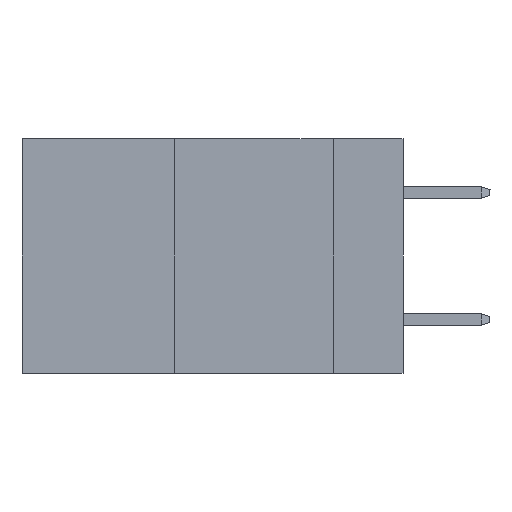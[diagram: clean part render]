
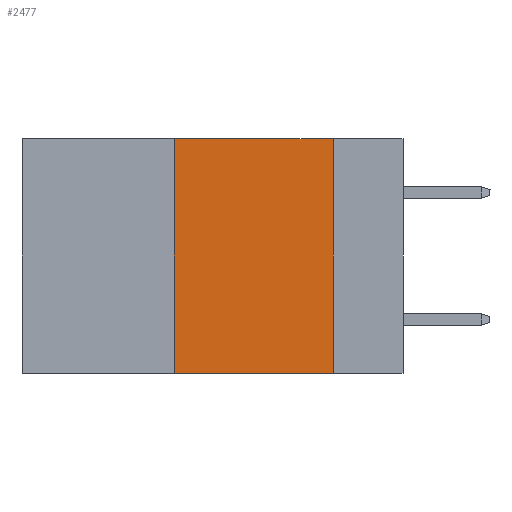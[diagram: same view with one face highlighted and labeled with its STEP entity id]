
A CAD part, left-side view. The second image highlights one B-rep face of the part: STEP entity #2477.
In plain terms, the highlighted planar face has unit normal (-1, 0, 0).
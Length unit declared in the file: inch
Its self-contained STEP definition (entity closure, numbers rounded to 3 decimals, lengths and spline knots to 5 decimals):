
#1628 = VERTEX_POINT ( 'NONE', #3738 ) ;
#1872 = EDGE_CURVE ( 'NONE', #18165, #4115, #6890, .T. ) ;
#2121 = ORIENTED_EDGE ( 'NONE', *, *, #6754, .F. ) ;
#2318 = EDGE_CURVE ( 'NONE', #18165, #10822, #6518, .T. ) ;
#2477 = ADVANCED_FACE ( 'NONE', ( #14035 ), #21450, .F. ) ;
#2865 = DIRECTION ( 'NONE',  ( 0., 0., -1. ) ) ;
#3508 = ORIENTED_EDGE ( 'NONE', *, *, #2318, .T. ) ;
#3557 = DIRECTION ( 'NONE',  ( 1., 0., 0. ) ) ;
#3738 = CARTESIAN_POINT ( 'NONE',  ( 0., 0.11, 0. ) ) ;
#4115 = VERTEX_POINT ( 'NONE', #4663 ) ;
#4663 = CARTESIAN_POINT ( 'NONE',  ( 0., 0.36, 0. ) ) ;
#4844 = LINE ( 'NONE', #12370, #21093 ) ;
#6518 = LINE ( 'NONE', #13802, #6992 ) ;
#6754 = EDGE_CURVE ( 'NONE', #4115, #1628, #4844, .T. ) ;
#6756 = VECTOR ( 'NONE', #2865, 39.37008 ) ;
#6890 = LINE ( 'NONE', #8611, #8922 ) ;
#6992 = VECTOR ( 'NONE', #17912, 39.37008 ) ;
#8611 = CARTESIAN_POINT ( 'NONE',  ( 0., 0.36, 0. ) ) ;
#8723 = DIRECTION ( 'NONE',  ( 0., 0., 1. ) ) ;
#8922 = VECTOR ( 'NONE', #8723, 39.37008 ) ;
#10822 = VERTEX_POINT ( 'NONE', #18458 ) ;
#10870 = AXIS2_PLACEMENT_3D ( 'NONE', #12212, #3557, #14873 ) ;
#10964 = ORIENTED_EDGE ( 'NONE', *, *, #15847, .F. ) ;
#12212 = CARTESIAN_POINT ( 'NONE',  ( 0., 0.6, 0. ) ) ;
#12370 = CARTESIAN_POINT ( 'NONE',  ( 0., 0.6, 0. ) ) ;
#13802 = CARTESIAN_POINT ( 'NONE',  ( 0., 0.6, -0.37 ) ) ;
#14035 = FACE_OUTER_BOUND ( 'NONE', #14654, .T. ) ;
#14654 = EDGE_LOOP ( 'NONE', ( #10964, #2121, #17548, #3508 ) ) ;
#14873 = DIRECTION ( 'NONE',  ( 0., 0., -1. ) ) ;
#15847 = EDGE_CURVE ( 'NONE', #1628, #10822, #21449, .T. ) ;
#17497 = DIRECTION ( 'NONE',  ( 0., -1., 0. ) ) ;
#17548 = ORIENTED_EDGE ( 'NONE', *, *, #1872, .F. ) ;
#17912 = DIRECTION ( 'NONE',  ( 0., -1., 0. ) ) ;
#18165 = VERTEX_POINT ( 'NONE', #19097 ) ;
#18458 = CARTESIAN_POINT ( 'NONE',  ( 0., 0.11, -0.37 ) ) ;
#19097 = CARTESIAN_POINT ( 'NONE',  ( 0., 0.36, -0.37 ) ) ;
#19509 = CARTESIAN_POINT ( 'NONE',  ( 0., 0.11, 0. ) ) ;
#21093 = VECTOR ( 'NONE', #17497, 39.37008 ) ;
#21449 = LINE ( 'NONE', #19509, #6756 ) ;
#21450 = PLANE ( 'NONE',  #10870 ) ;
